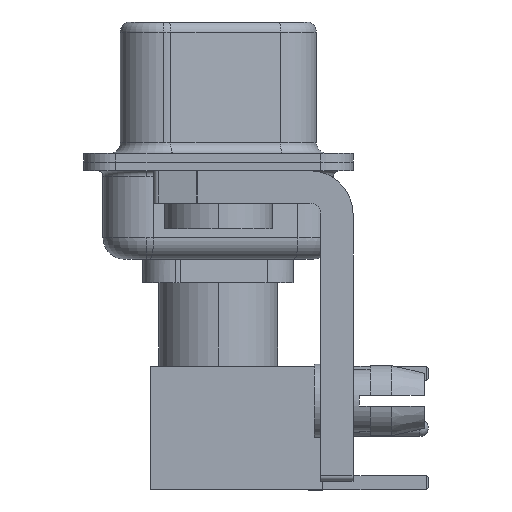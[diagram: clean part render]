
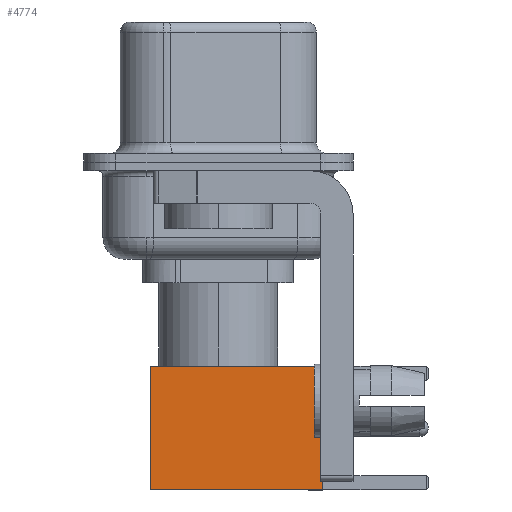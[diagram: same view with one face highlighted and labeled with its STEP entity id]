
A CAD part, left-side view. The second image highlights one B-rep face of the part: STEP entity #4774.
In plain terms, the highlighted face is planar.
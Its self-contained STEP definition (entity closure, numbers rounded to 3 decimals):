
#840 = LINE ( 'NONE', #13305, #15222 ) ;
#1086 = CARTESIAN_POINT ( 'NONE',  ( 2.875, 2.875, 0. ) ) ;
#1439 = VECTOR ( 'NONE', #9702, 1000. ) ;
#1780 = VERTEX_POINT ( 'NONE', #13767 ) ;
#2872 = CARTESIAN_POINT ( 'NONE',  ( -2.875, 2.875, 0. ) ) ;
#3211 = CARTESIAN_POINT ( 'NONE',  ( 2.875, 2.875, 0. ) ) ;
#3536 = VECTOR ( 'NONE', #13543, 1000. ) ;
#4375 = AXIS2_PLACEMENT_3D ( 'NONE', #17894, #11876, #18101 ) ;
#4774 = ADVANCED_FACE ( 'NONE', ( #11672 ), #7202, .T. ) ;
#5376 = DIRECTION ( 'NONE',  ( 0., 0., -1. ) ) ;
#5718 = EDGE_CURVE ( 'NONE', #1780, #13949, #8865, .T. ) ;
#7202 = PLANE ( 'NONE',  #4375 ) ;
#7264 = LINE ( 'NONE', #8882, #19621 ) ;
#7929 = VERTEX_POINT ( 'NONE', #12360 ) ;
#8865 = LINE ( 'NONE', #1086, #3536 ) ;
#8882 = CARTESIAN_POINT ( 'NONE',  ( 0., 2.875, 0. ) ) ;
#9229 = ORIENTED_EDGE ( 'NONE', *, *, #10307, .F. ) ;
#9702 = DIRECTION ( 'NONE',  ( -1., 0., 0. ) ) ;
#9898 = CARTESIAN_POINT ( 'NONE',  ( 0., 2.875, 8. ) ) ;
#10307 = EDGE_CURVE ( 'NONE', #1780, #7929, #11537, .T. ) ;
#10556 = EDGE_CURVE ( 'NONE', #13949, #11183, #7264, .T. ) ;
#11183 = VERTEX_POINT ( 'NONE', #2872 ) ;
#11537 = LINE ( 'NONE', #9898, #1439 ) ;
#11672 = FACE_OUTER_BOUND ( 'NONE', #14347, .T. ) ;
#11876 = DIRECTION ( 'NONE',  ( 0., 1., 0. ) ) ;
#12360 = CARTESIAN_POINT ( 'NONE',  ( -2.875, 2.875, 8. ) ) ;
#12519 = ORIENTED_EDGE ( 'NONE', *, *, #16654, .F. ) ;
#13305 = CARTESIAN_POINT ( 'NONE',  ( -2.875, 2.875, 0. ) ) ;
#13543 = DIRECTION ( 'NONE',  ( 0., 0., -1. ) ) ;
#13767 = CARTESIAN_POINT ( 'NONE',  ( 2.875, 2.875, 8. ) ) ;
#13949 = VERTEX_POINT ( 'NONE', #3211 ) ;
#14347 = EDGE_LOOP ( 'NONE', ( #17971, #18366, #12519, #9229 ) ) ;
#15101 = DIRECTION ( 'NONE',  ( -1., 0., 0. ) ) ;
#15222 = VECTOR ( 'NONE', #5376, 1000. ) ;
#16654 = EDGE_CURVE ( 'NONE', #7929, #11183, #840, .T. ) ;
#17894 = CARTESIAN_POINT ( 'NONE',  ( 2.875, 2.875, 0. ) ) ;
#17971 = ORIENTED_EDGE ( 'NONE', *, *, #5718, .T. ) ;
#18101 = DIRECTION ( 'NONE',  ( 0., 0., 1. ) ) ;
#18366 = ORIENTED_EDGE ( 'NONE', *, *, #10556, .T. ) ;
#19621 = VECTOR ( 'NONE', #15101, 1000. ) ;
